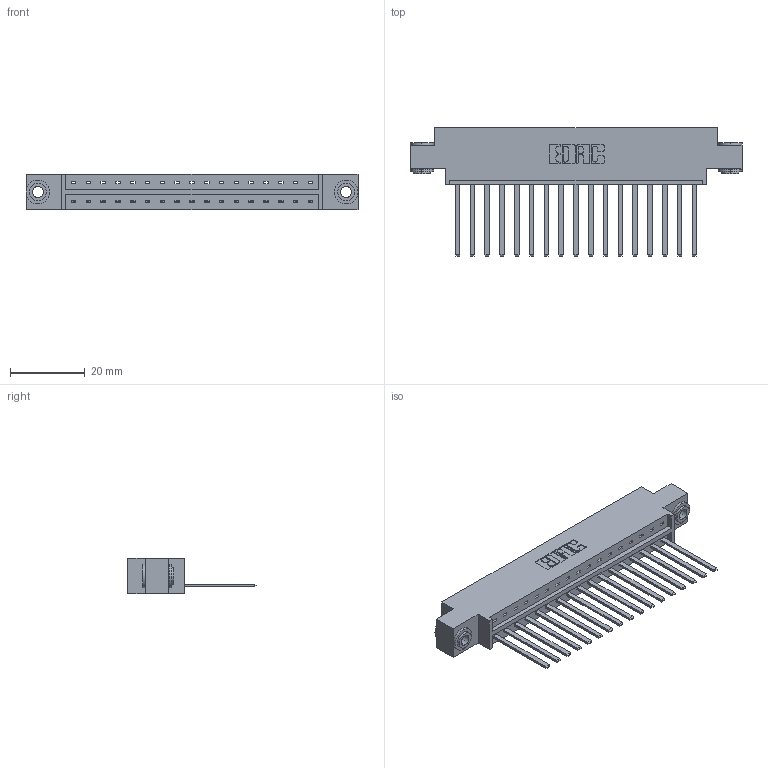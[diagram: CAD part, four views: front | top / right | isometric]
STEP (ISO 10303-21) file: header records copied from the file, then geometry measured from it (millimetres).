
FILE_DESCRIPTION (( 'STEP AP203' ), '1' );
FILE_NAME ('333-017-544-603.STEP', '2019-08-09T12:16:36', ( '' ), ( '' ), 'SwSTEP 2.0', 'SolidWorks 2016', '' );
FILE_SCHEMA (( 'CONFIG_CONTROL_DESIGN' ));
Length unit declared in the file: inch
Products named in the file (4): 333 Part_Offset - .156 Dia - TH; 333-017-544-603; 345-250-002_345-250-002-102; 345-292-001_345-293-144
Assembly tree (20 placements, depth 2):
  333-017-544-603
    333 Part_Offset - .156 Dia - TH
    345-292-001_345-293-144  x17
    345-250-002_345-250-002-102  x2
Bounding box: 88.9 x 34.3 x 9.4 mm (x, y, z)
Volume: 8719.3 mm3; surface area: 10336.3 mm2
Topology: 20 solids, 20 shells, 1040 faces, 3085 edges, 2030 vertices
Faces by surface type: plane 730, cylinder 302, cone 8
Entity records: 14224 total; most frequent: CARTESIAN_POINT 2436, ORIENTED_EDGE 2382, DIRECTION 2135, EDGE_CURVE 1191, VECTOR 1043, LINE 1043, VERTEX_POINT 790, AXIS2_PLACEMENT_3D 546
